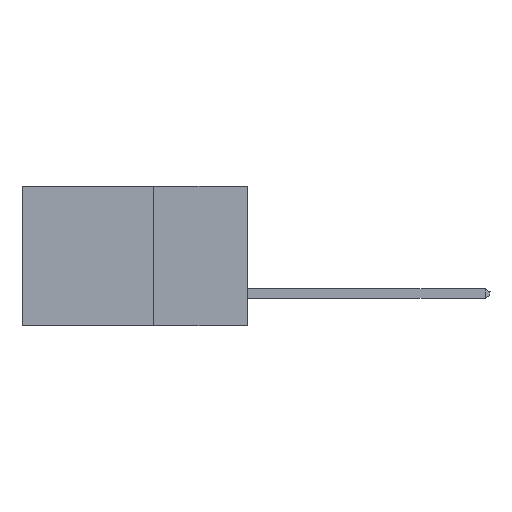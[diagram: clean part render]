
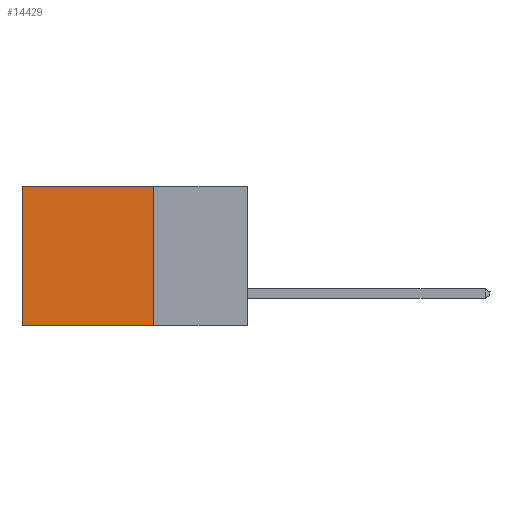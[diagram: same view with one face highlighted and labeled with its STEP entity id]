
A CAD part, left-side view. The second image highlights one B-rep face of the part: STEP entity #14429.
In plain terms, the highlighted planar face has unit normal (-1, 0, 0).
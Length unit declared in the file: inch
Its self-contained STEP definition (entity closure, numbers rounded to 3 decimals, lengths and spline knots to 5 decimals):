
#645 = VERTEX_POINT ( 'NONE', #5521 ) ;
#1034 = LINE ( 'NONE', #15993, #14439 ) ;
#2088 = EDGE_CURVE ( 'NONE', #645, #5328, #1034, .T. ) ;
#2314 = DIRECTION ( 'NONE',  ( 0., 0., -1. ) ) ;
#2890 = DIRECTION ( 'NONE',  ( 0., 0., -1. ) ) ;
#3650 = EDGE_CURVE ( 'NONE', #9505, #5328, #6808, .T. ) ;
#3852 = VERTEX_POINT ( 'NONE', #11084 ) ;
#4367 = PLANE ( 'NONE',  #9122 ) ;
#5190 = EDGE_CURVE ( 'NONE', #3852, #9505, #12701, .T. ) ;
#5328 = VERTEX_POINT ( 'NONE', #11161 ) ;
#5521 = CARTESIAN_POINT ( 'NONE',  ( 0.2615, 0.25, -0.37 ) ) ;
#6127 = DIRECTION ( 'NONE',  ( 0., 0., -1. ) ) ;
#6732 = CARTESIAN_POINT ( 'NONE',  ( 0.2615, 0.25, -0.37 ) ) ;
#6808 = LINE ( 'NONE', #15320, #10690 ) ;
#7144 = DIRECTION ( 'NONE',  ( 0., 1., 0. ) ) ;
#7192 = FACE_OUTER_BOUND ( 'NONE', #15564, .T. ) ;
#9122 = AXIS2_PLACEMENT_3D ( 'NONE', #6732, #13438, #2314 ) ;
#9292 = ORIENTED_EDGE ( 'NONE', *, *, #3650, .T. ) ;
#9505 = VERTEX_POINT ( 'NONE', #9821 ) ;
#9821 = CARTESIAN_POINT ( 'NONE',  ( 0.2615, 0.6, 0. ) ) ;
#9951 = DIRECTION ( 'NONE',  ( 0., 1., 0. ) ) ;
#10414 = EDGE_CURVE ( 'NONE', #3852, #645, #13504, .T. ) ;
#10690 = VECTOR ( 'NONE', #2890, 39.37008 ) ;
#11084 = CARTESIAN_POINT ( 'NONE',  ( 0.2615, 0.25, 0. ) ) ;
#11161 = CARTESIAN_POINT ( 'NONE',  ( 0.2615, 0.6, -0.37 ) ) ;
#11171 = ORIENTED_EDGE ( 'NONE', *, *, #10414, .F. ) ;
#11285 = VECTOR ( 'NONE', #9951, 39.37008 ) ;
#11314 = CARTESIAN_POINT ( 'NONE',  ( 0.2615, 0.25, 0. ) ) ;
#12278 = CARTESIAN_POINT ( 'NONE',  ( 0.2615, 0.25, -0.37 ) ) ;
#12403 = VECTOR ( 'NONE', #6127, 39.37008 ) ;
#12701 = LINE ( 'NONE', #11314, #11285 ) ;
#12989 = ORIENTED_EDGE ( 'NONE', *, *, #2088, .F. ) ;
#13438 = DIRECTION ( 'NONE',  ( 1., 0., 0. ) ) ;
#13504 = LINE ( 'NONE', #12278, #12403 ) ;
#14190 = ORIENTED_EDGE ( 'NONE', *, *, #5190, .T. ) ;
#14429 = ADVANCED_FACE ( 'NONE', ( #7192 ), #4367, .F. ) ;
#14439 = VECTOR ( 'NONE', #7144, 39.37008 ) ;
#15320 = CARTESIAN_POINT ( 'NONE',  ( 0.2615, 0.6, -0.37 ) ) ;
#15564 = EDGE_LOOP ( 'NONE', ( #9292, #12989, #11171, #14190 ) ) ;
#15993 = CARTESIAN_POINT ( 'NONE',  ( 0.2615, 0.25, -0.37 ) ) ;
